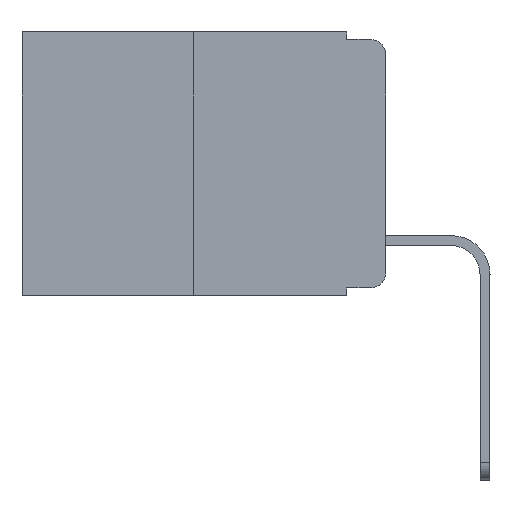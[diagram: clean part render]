
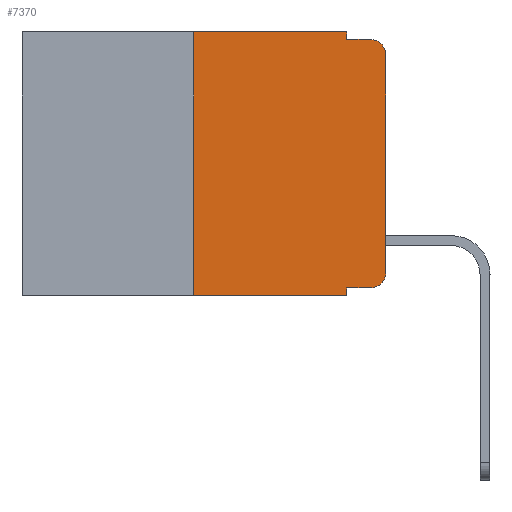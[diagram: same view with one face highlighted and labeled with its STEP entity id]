
A CAD part, left-side view. The second image highlights one B-rep face of the part: STEP entity #7370.
In plain terms, the highlighted planar face has unit normal (-1, 0, 0).
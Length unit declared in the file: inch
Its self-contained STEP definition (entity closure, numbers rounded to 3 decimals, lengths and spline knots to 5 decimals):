
#340 = VERTEX_POINT ( 'NONE', #5920 ) ;
#380 = EDGE_CURVE ( 'NONE', #4790, #405, #4075, .T. ) ;
#385 = ORIENTED_EDGE ( 'NONE', *, *, #4729, .F. ) ;
#405 = VERTEX_POINT ( 'NONE', #9726 ) ;
#446 = DIRECTION ( 'NONE',  ( 0., -1., 0. ) ) ;
#529 = EDGE_CURVE ( 'NONE', #9642, #340, #6806, .T. ) ;
#682 = DIRECTION ( 'NONE',  ( 0., 0., -1. ) ) ;
#696 = AXIS2_PLACEMENT_3D ( 'NONE', #11314, #11437, #10510 ) ;
#751 = VERTEX_POINT ( 'NONE', #10036 ) ;
#775 = VECTOR ( 'NONE', #446, 39.37008 ) ;
#856 = VECTOR ( 'NONE', #8682, 39.37008 ) ;
#1035 = EDGE_LOOP ( 'NONE', ( #10531, #11474, #2449, #10951, #2911, #4083, #7796, #385, #5639, #9601 ) ) ;
#1173 = VERTEX_POINT ( 'NONE', #4284 ) ;
#1447 = CARTESIAN_POINT ( 'NONE',  ( 0., 0.051, -0.333 ) ) ;
#1522 = CARTESIAN_POINT ( 'NONE',  ( 0., 0.051, -0.343 ) ) ;
#1561 = CARTESIAN_POINT ( 'NONE',  ( 0., 0.051, -0.01 ) ) ;
#1696 = CARTESIAN_POINT ( 'NONE',  ( 0., 0., 0. ) ) ;
#1735 = VECTOR ( 'NONE', #6719, 39.37008 ) ;
#1891 = VECTOR ( 'NONE', #8848, 39.37008 ) ;
#2159 = PLANE ( 'NONE',  #696 ) ;
#2392 = EDGE_CURVE ( 'NONE', #340, #751, #6147, .T. ) ;
#2449 = ORIENTED_EDGE ( 'NONE', *, *, #380, .F. ) ;
#2692 = EDGE_CURVE ( 'NONE', #4102, #9535, #10901, .T. ) ;
#2727 = CARTESIAN_POINT ( 'NONE',  ( 0., 0.02, -0.333 ) ) ;
#2903 = VECTOR ( 'NONE', #7769, 39.37008 ) ;
#2911 = ORIENTED_EDGE ( 'NONE', *, *, #2692, .F. ) ;
#2994 = AXIS2_PLACEMENT_3D ( 'NONE', #5118, #6839, #10583 ) ;
#3056 = LINE ( 'NONE', #3273, #2903 ) ;
#3165 = FACE_OUTER_BOUND ( 'NONE', #1035, .T. ) ;
#3226 = VERTEX_POINT ( 'NONE', #1447 ) ;
#3273 = CARTESIAN_POINT ( 'NONE',  ( 0., 0.051, -0.333 ) ) ;
#3812 = LINE ( 'NONE', #6079, #6239 ) ;
#4075 = LINE ( 'NONE', #10666, #6527 ) ;
#4083 = ORIENTED_EDGE ( 'NONE', *, *, #7842, .F. ) ;
#4102 = VERTEX_POINT ( 'NONE', #11326 ) ;
#4198 = CIRCLE ( 'NONE', #2994, 0.02 ) ;
#4284 = CARTESIAN_POINT ( 'NONE',  ( 0., 0.25, -0.343 ) ) ;
#4358 = DIRECTION ( 'NONE',  ( 0., 0., -1. ) ) ;
#4504 = AXIS2_PLACEMENT_3D ( 'NONE', #9089, #5233, #4358 ) ;
#4729 = EDGE_CURVE ( 'NONE', #3226, #6693, #3812, .T. ) ;
#4790 = VERTEX_POINT ( 'NONE', #1561 ) ;
#5118 = CARTESIAN_POINT ( 'NONE',  ( 0., 0.02, -0.03 ) ) ;
#5233 = DIRECTION ( 'NONE',  ( -1., 0., 0. ) ) ;
#5299 = EDGE_CURVE ( 'NONE', #751, #405, #4198, .T. ) ;
#5639 = ORIENTED_EDGE ( 'NONE', *, *, #8691, .T. ) ;
#5821 = CARTESIAN_POINT ( 'NONE',  ( 0., 0.473, -0.343 ) ) ;
#5906 = EDGE_CURVE ( 'NONE', #1173, #6693, #8663, .T. ) ;
#5920 = CARTESIAN_POINT ( 'NONE',  ( 0., 0., -0.313 ) ) ;
#5973 = CARTESIAN_POINT ( 'NONE',  ( 0., 0.051, 0. ) ) ;
#6007 = EDGE_CURVE ( 'NONE', #9535, #4790, #11381, .T. ) ;
#6079 = CARTESIAN_POINT ( 'NONE',  ( 0., 0.051, 0. ) ) ;
#6147 = LINE ( 'NONE', #1696, #7163 ) ;
#6239 = VECTOR ( 'NONE', #682, 39.37008 ) ;
#6527 = VECTOR ( 'NONE', #9807, 39.37008 ) ;
#6693 = VERTEX_POINT ( 'NONE', #1522 ) ;
#6719 = DIRECTION ( 'NONE',  ( 0., 0., 1. ) ) ;
#6806 = CIRCLE ( 'NONE', #4504, 0.02 ) ;
#6839 = DIRECTION ( 'NONE',  ( -1., 0., 0. ) ) ;
#7163 = VECTOR ( 'NONE', #8097, 39.37008 ) ;
#7370 = ADVANCED_FACE ( 'NONE', ( #3165 ), #2159, .F. ) ;
#7769 = DIRECTION ( 'NONE',  ( 0., -1., 0. ) ) ;
#7796 = ORIENTED_EDGE ( 'NONE', *, *, #5906, .T. ) ;
#7842 = EDGE_CURVE ( 'NONE', #1173, #4102, #8337, .T. ) ;
#8097 = DIRECTION ( 'NONE',  ( 0., 0., 1. ) ) ;
#8123 = CARTESIAN_POINT ( 'NONE',  ( 0., 0.051, 0. ) ) ;
#8337 = LINE ( 'NONE', #11216, #1735 ) ;
#8559 = CARTESIAN_POINT ( 'NONE',  ( 0., 0.473, 0. ) ) ;
#8663 = LINE ( 'NONE', #5821, #775 ) ;
#8682 = DIRECTION ( 'NONE',  ( 0., -1., 0. ) ) ;
#8691 = EDGE_CURVE ( 'NONE', #3226, #9642, #3056, .T. ) ;
#8848 = DIRECTION ( 'NONE',  ( 0., 0., -1. ) ) ;
#9089 = CARTESIAN_POINT ( 'NONE',  ( 0., 0.02, -0.313 ) ) ;
#9535 = VERTEX_POINT ( 'NONE', #8123 ) ;
#9601 = ORIENTED_EDGE ( 'NONE', *, *, #529, .T. ) ;
#9642 = VERTEX_POINT ( 'NONE', #2727 ) ;
#9726 = CARTESIAN_POINT ( 'NONE',  ( 0., 0.02, -0.01 ) ) ;
#9807 = DIRECTION ( 'NONE',  ( 0., -1., 0. ) ) ;
#10036 = CARTESIAN_POINT ( 'NONE',  ( 0., 0., -0.03 ) ) ;
#10510 = DIRECTION ( 'NONE',  ( 0., 0., -1. ) ) ;
#10531 = ORIENTED_EDGE ( 'NONE', *, *, #2392, .T. ) ;
#10583 = DIRECTION ( 'NONE',  ( 0., 0., -1. ) ) ;
#10666 = CARTESIAN_POINT ( 'NONE',  ( 0., 0.051, -0.01 ) ) ;
#10901 = LINE ( 'NONE', #8559, #856 ) ;
#10951 = ORIENTED_EDGE ( 'NONE', *, *, #6007, .F. ) ;
#11216 = CARTESIAN_POINT ( 'NONE',  ( 0., 0.25, 0. ) ) ;
#11314 = CARTESIAN_POINT ( 'NONE',  ( 0., 0.473, 0. ) ) ;
#11326 = CARTESIAN_POINT ( 'NONE',  ( 0., 0.25, 0. ) ) ;
#11381 = LINE ( 'NONE', #5973, #1891 ) ;
#11437 = DIRECTION ( 'NONE',  ( 1., 0., 0. ) ) ;
#11474 = ORIENTED_EDGE ( 'NONE', *, *, #5299, .T. ) ;
